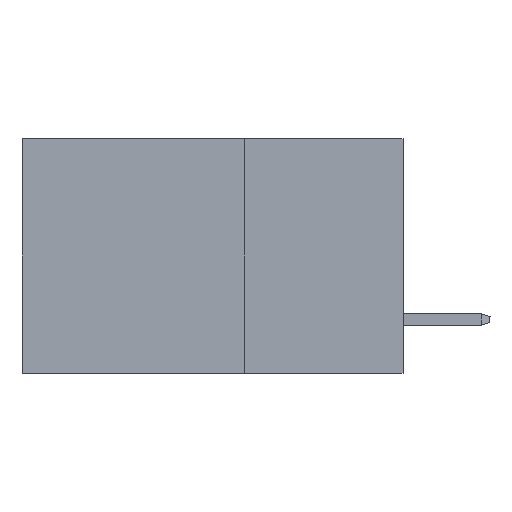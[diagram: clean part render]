
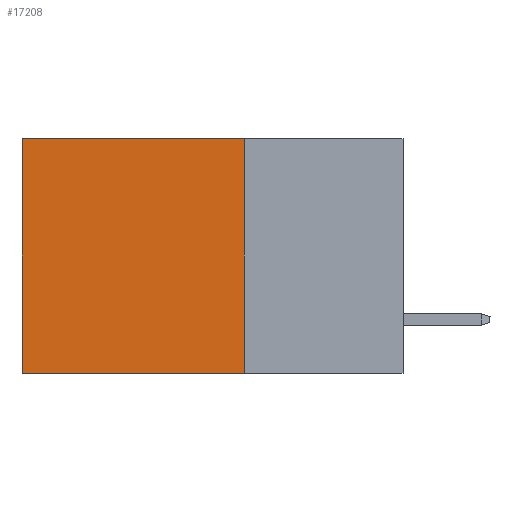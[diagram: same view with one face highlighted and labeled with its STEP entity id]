
A CAD part, left-side view. The second image highlights one B-rep face of the part: STEP entity #17208.
In plain terms, the highlighted planar face has unit normal (-1, 0, 0).
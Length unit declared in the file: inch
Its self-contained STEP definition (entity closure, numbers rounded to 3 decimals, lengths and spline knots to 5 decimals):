
#8 = CARTESIAN_POINT ( 'NONE',  ( 0.2875, 0.6, -0.37 ) ) ;
#2421 = CARTESIAN_POINT ( 'NONE',  ( 0.2875, 0.25, -0.37 ) ) ;
#3029 = DIRECTION ( 'NONE',  ( 0., 1., 0. ) ) ;
#3081 = DIRECTION ( 'NONE',  ( 0., 0., -1. ) ) ;
#4947 = LINE ( 'NONE', #23284, #13012 ) ;
#5572 = VERTEX_POINT ( 'NONE', #8 ) ;
#6378 = CARTESIAN_POINT ( 'NONE',  ( 0.2875, 0.25, 0. ) ) ;
#6588 = AXIS2_PLACEMENT_3D ( 'NONE', #14958, #23663, #3081 ) ;
#8088 = LINE ( 'NONE', #6378, #9695 ) ;
#8940 = VERTEX_POINT ( 'NONE', #24281 ) ;
#9033 = DIRECTION ( 'NONE',  ( 0., 0., -1. ) ) ;
#9284 = ORIENTED_EDGE ( 'NONE', *, *, #23777, .F. ) ;
#9695 = VECTOR ( 'NONE', #18524, 39.37008 ) ;
#9738 = VERTEX_POINT ( 'NONE', #23438 ) ;
#10609 = PLANE ( 'NONE',  #6588 ) ;
#11208 = LINE ( 'NONE', #21127, #11277 ) ;
#11277 = VECTOR ( 'NONE', #3029, 39.37008 ) ;
#12850 = DIRECTION ( 'NONE',  ( 0., 1., 0. ) ) ;
#13012 = VECTOR ( 'NONE', #9033, 39.37008 ) ;
#14195 = ORIENTED_EDGE ( 'NONE', *, *, #22272, .T. ) ;
#14640 = VECTOR ( 'NONE', #12850, 39.37008 ) ;
#14958 = CARTESIAN_POINT ( 'NONE',  ( 0.2875, 0.25, 0. ) ) ;
#17208 = ADVANCED_FACE ( 'NONE', ( #20654 ), #10609, .F. ) ;
#17700 = ORIENTED_EDGE ( 'NONE', *, *, #20643, .T. ) ;
#18340 = EDGE_CURVE ( 'NONE', #8940, #5572, #20523, .T. ) ;
#18524 = DIRECTION ( 'NONE',  ( 0., 0., -1. ) ) ;
#18661 = VERTEX_POINT ( 'NONE', #22872 ) ;
#19839 = EDGE_LOOP ( 'NONE', ( #14195, #20719, #9284, #17700 ) ) ;
#20523 = LINE ( 'NONE', #2421, #14640 ) ;
#20643 = EDGE_CURVE ( 'NONE', #18661, #9738, #11208, .T. ) ;
#20654 = FACE_OUTER_BOUND ( 'NONE', #19839, .T. ) ;
#20719 = ORIENTED_EDGE ( 'NONE', *, *, #18340, .F. ) ;
#21127 = CARTESIAN_POINT ( 'NONE',  ( 0.2875, 0.25, 0. ) ) ;
#22272 = EDGE_CURVE ( 'NONE', #9738, #5572, #4947, .T. ) ;
#22872 = CARTESIAN_POINT ( 'NONE',  ( 0.2875, 0.25, 0. ) ) ;
#23284 = CARTESIAN_POINT ( 'NONE',  ( 0.2875, 0.6, 0. ) ) ;
#23438 = CARTESIAN_POINT ( 'NONE',  ( 0.2875, 0.6, 0. ) ) ;
#23663 = DIRECTION ( 'NONE',  ( 1., 0., 0. ) ) ;
#23777 = EDGE_CURVE ( 'NONE', #18661, #8940, #8088, .T. ) ;
#24281 = CARTESIAN_POINT ( 'NONE',  ( 0.2875, 0.25, -0.37 ) ) ;
